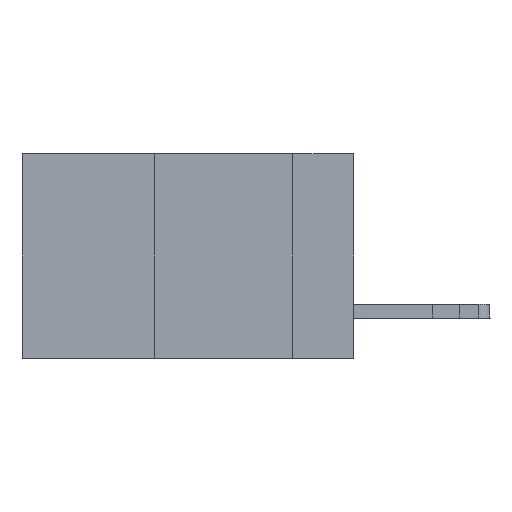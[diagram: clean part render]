
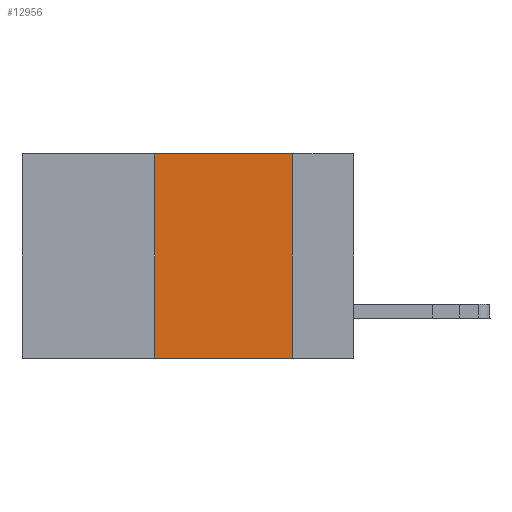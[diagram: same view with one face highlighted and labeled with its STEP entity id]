
A CAD part, left-side view. The second image highlights one B-rep face of the part: STEP entity #12956.
In plain terms, the highlighted planar face has unit normal (-1, 0, 0).
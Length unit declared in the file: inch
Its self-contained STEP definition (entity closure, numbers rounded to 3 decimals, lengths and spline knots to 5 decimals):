
#37 = VERTEX_POINT ( 'NONE', #3629 ) ;
#63 = VECTOR ( 'NONE', #14057, 39.37008 ) ;
#562 = FACE_OUTER_BOUND ( 'NONE', #11168, .T. ) ;
#1308 = CARTESIAN_POINT ( 'NONE',  ( 0., 0.6, 0. ) ) ;
#1729 = DIRECTION ( 'NONE',  ( 0., 0., -1. ) ) ;
#2501 = CARTESIAN_POINT ( 'NONE',  ( 0., 0.11, 0. ) ) ;
#2704 = ORIENTED_EDGE ( 'NONE', *, *, #3570, .T. ) ;
#3570 = EDGE_CURVE ( 'NONE', #5458, #14958, #7487, .T. ) ;
#3629 = CARTESIAN_POINT ( 'NONE',  ( 0., 0.36, 0. ) ) ;
#3754 = EDGE_CURVE ( 'NONE', #37, #12767, #15451, .T. ) ;
#4045 = VECTOR ( 'NONE', #15772, 39.37008 ) ;
#4060 = VECTOR ( 'NONE', #9108, 39.37008 ) ;
#4650 = VECTOR ( 'NONE', #9683, 39.37008 ) ;
#5395 = CARTESIAN_POINT ( 'NONE',  ( 0., 0.6, -0.37 ) ) ;
#5458 = VERTEX_POINT ( 'NONE', #8520 ) ;
#7123 = AXIS2_PLACEMENT_3D ( 'NONE', #10852, #9603, #1729 ) ;
#7487 = LINE ( 'NONE', #5395, #4045 ) ;
#7503 = LINE ( 'NONE', #2501, #4060 ) ;
#8520 = CARTESIAN_POINT ( 'NONE',  ( 0., 0.36, -0.37 ) ) ;
#9108 = DIRECTION ( 'NONE',  ( 0., 0., -1. ) ) ;
#9286 = ORIENTED_EDGE ( 'NONE', *, *, #12021, .F. ) ;
#9603 = DIRECTION ( 'NONE',  ( 1., 0., 0. ) ) ;
#9683 = DIRECTION ( 'NONE',  ( 0., -1., 0. ) ) ;
#10611 = LINE ( 'NONE', #12814, #63 ) ;
#10852 = CARTESIAN_POINT ( 'NONE',  ( 0., 0.6, 0. ) ) ;
#11168 = EDGE_LOOP ( 'NONE', ( #9286, #16551, #11693, #2704 ) ) ;
#11693 = ORIENTED_EDGE ( 'NONE', *, *, #13793, .F. ) ;
#12021 = EDGE_CURVE ( 'NONE', #12767, #14958, #7503, .T. ) ;
#12767 = VERTEX_POINT ( 'NONE', #15630 ) ;
#12814 = CARTESIAN_POINT ( 'NONE',  ( 0., 0.36, 0. ) ) ;
#12956 = ADVANCED_FACE ( 'NONE', ( #562 ), #14800, .F. ) ;
#13793 = EDGE_CURVE ( 'NONE', #5458, #37, #10611, .T. ) ;
#14057 = DIRECTION ( 'NONE',  ( 0., 0., 1. ) ) ;
#14800 = PLANE ( 'NONE',  #7123 ) ;
#14863 = CARTESIAN_POINT ( 'NONE',  ( 0., 0.11, -0.37 ) ) ;
#14958 = VERTEX_POINT ( 'NONE', #14863 ) ;
#15451 = LINE ( 'NONE', #1308, #4650 ) ;
#15630 = CARTESIAN_POINT ( 'NONE',  ( 0., 0.11, 0. ) ) ;
#15772 = DIRECTION ( 'NONE',  ( 0., -1., 0. ) ) ;
#16551 = ORIENTED_EDGE ( 'NONE', *, *, #3754, .F. ) ;
